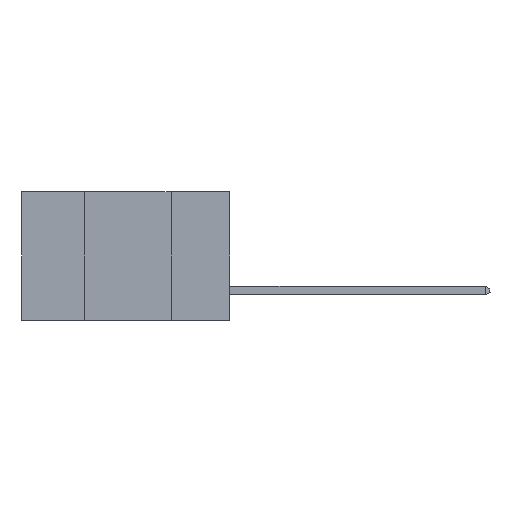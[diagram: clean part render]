
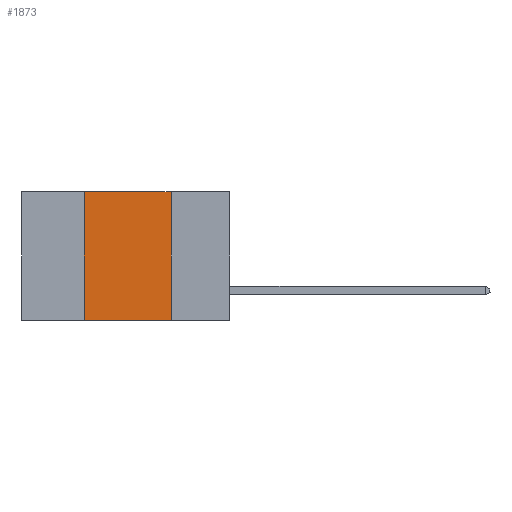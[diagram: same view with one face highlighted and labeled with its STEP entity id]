
A CAD part, left-side view. The second image highlights one B-rep face of the part: STEP entity #1873.
In plain terms, the highlighted planar face has unit normal (-1, 0, 0).
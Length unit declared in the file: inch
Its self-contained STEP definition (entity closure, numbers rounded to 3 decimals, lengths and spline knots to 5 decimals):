
#71 = ORIENTED_EDGE ( 'NONE', *, *, #4166, .F. ) ;
#1873 = ADVANCED_FACE ( 'NONE', ( #17271 ), #11779, .F. ) ;
#1942 = VERTEX_POINT ( 'NONE', #17452 ) ;
#2357 = CARTESIAN_POINT ( 'NONE',  ( 0., 0.6, 0. ) ) ;
#3069 = DIRECTION ( 'NONE',  ( 0., 0., 1. ) ) ;
#3192 = AXIS2_PLACEMENT_3D ( 'NONE', #2357, #21435, #7066 ) ;
#4166 = EDGE_CURVE ( 'NONE', #30881, #19861, #24969, .T. ) ;
#5614 = VECTOR ( 'NONE', #3069, 39.37008 ) ;
#6986 = VECTOR ( 'NONE', #13639, 39.37008 ) ;
#7066 = DIRECTION ( 'NONE',  ( 0., 0., -1. ) ) ;
#10738 = DIRECTION ( 'NONE',  ( 0., -1., 0. ) ) ;
#10779 = VECTOR ( 'NONE', #10738, 39.37008 ) ;
#11779 = PLANE ( 'NONE',  #3192 ) ;
#12023 = EDGE_CURVE ( 'NONE', #28516, #30881, #27364, .T. ) ;
#13070 = CARTESIAN_POINT ( 'NONE',  ( 0., 0.6, -0.37 ) ) ;
#13639 = DIRECTION ( 'NONE',  ( 0., -1., 0. ) ) ;
#13676 = VECTOR ( 'NONE', #31047, 39.37008 ) ;
#13903 = EDGE_LOOP ( 'NONE', ( #23005, #71, #17634, #19967 ) ) ;
#16281 = CARTESIAN_POINT ( 'NONE',  ( 0., 0.17, 0. ) ) ;
#17271 = FACE_OUTER_BOUND ( 'NONE', #13903, .T. ) ;
#17452 = CARTESIAN_POINT ( 'NONE',  ( 0., 0.17, -0.37 ) ) ;
#17634 = ORIENTED_EDGE ( 'NONE', *, *, #12023, .F. ) ;
#17703 = CARTESIAN_POINT ( 'NONE',  ( 0., 0.42, 0. ) ) ;
#19861 = VERTEX_POINT ( 'NONE', #24016 ) ;
#19967 = ORIENTED_EDGE ( 'NONE', *, *, #31023, .T. ) ;
#20085 = CARTESIAN_POINT ( 'NONE',  ( 0., 0.42, -0.37 ) ) ;
#20175 = LINE ( 'NONE', #13070, #10779 ) ;
#21435 = DIRECTION ( 'NONE',  ( 1., 0., 0. ) ) ;
#22415 = CARTESIAN_POINT ( 'NONE',  ( 0., 0.42, 0. ) ) ;
#23005 = ORIENTED_EDGE ( 'NONE', *, *, #25592, .F. ) ;
#24016 = CARTESIAN_POINT ( 'NONE',  ( 0., 0.17, 0. ) ) ;
#24969 = LINE ( 'NONE', #30399, #6986 ) ;
#25592 = EDGE_CURVE ( 'NONE', #19861, #1942, #29022, .T. ) ;
#27364 = LINE ( 'NONE', #22415, #5614 ) ;
#28516 = VERTEX_POINT ( 'NONE', #20085 ) ;
#29022 = LINE ( 'NONE', #16281, #13676 ) ;
#30399 = CARTESIAN_POINT ( 'NONE',  ( 0., 0.6, 0. ) ) ;
#30881 = VERTEX_POINT ( 'NONE', #17703 ) ;
#31023 = EDGE_CURVE ( 'NONE', #28516, #1942, #20175, .T. ) ;
#31047 = DIRECTION ( 'NONE',  ( 0., 0., -1. ) ) ;
